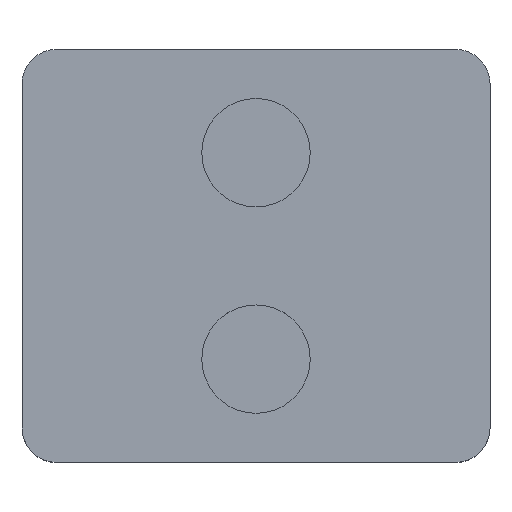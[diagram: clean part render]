
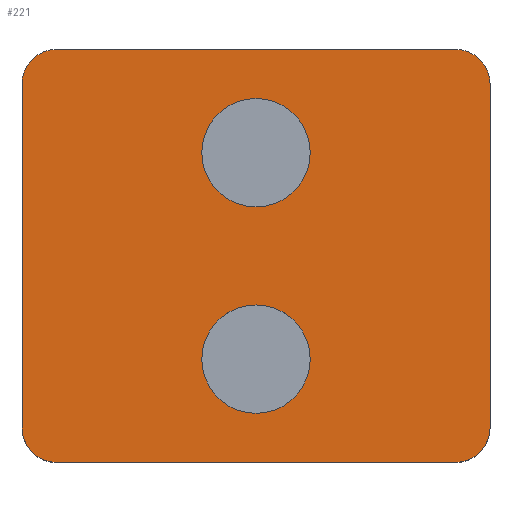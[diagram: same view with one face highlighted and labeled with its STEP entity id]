
A CAD part, top view. The second image highlights one B-rep face of the part: STEP entity #221.
In plain terms, the highlighted planar face has unit normal (0, 0, 1).
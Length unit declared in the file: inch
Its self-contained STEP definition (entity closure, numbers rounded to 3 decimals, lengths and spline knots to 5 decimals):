
#15=FACE_BOUND('',#42,.T.);
#16=FACE_BOUND('',#43,.T.);
#18=PLANE('',#251);
#27=FACE_OUTER_BOUND('',#41,.T.);
#41=EDGE_LOOP('',(#161,#162,#163,#164,#165,#166,#167,#168));
#42=EDGE_LOOP('',(#169));
#43=EDGE_LOOP('',(#170));
#57=LINE('',#357,#75);
#60=LINE('',#363,#78);
#61=LINE('',#367,#79);
#62=LINE('',#371,#80);
#75=VECTOR('',#285,0.3937);
#78=VECTOR('',#290,0.3937);
#79=VECTOR('',#293,0.3937);
#80=VECTOR('',#296,0.3937);
#92=CIRCLE('',#249,0.0625);
#93=CIRCLE('',#252,0.0625);
#94=CIRCLE('',#253,0.0625);
#95=CIRCLE('',#254,0.0625);
#96=CIRCLE('',#255,0.09843);
#97=CIRCLE('',#256,0.09843);
#105=VERTEX_POINT('',#350);
#106=VERTEX_POINT('',#352);
#107=VERTEX_POINT('',#356);
#109=VERTEX_POINT('',#362);
#110=VERTEX_POINT('',#364);
#111=VERTEX_POINT('',#366);
#112=VERTEX_POINT('',#368);
#113=VERTEX_POINT('',#370);
#114=VERTEX_POINT('',#373);
#115=VERTEX_POINT('',#375);
#125=EDGE_CURVE('',#105,#106,#92,.T.);
#127=EDGE_CURVE('',#107,#106,#57,.T.);
#130=EDGE_CURVE('',#105,#109,#60,.T.);
#131=EDGE_CURVE('',#110,#109,#93,.T.);
#132=EDGE_CURVE('',#110,#111,#61,.T.);
#133=EDGE_CURVE('',#112,#111,#94,.T.);
#134=EDGE_CURVE('',#112,#113,#62,.T.);
#135=EDGE_CURVE('',#107,#113,#95,.T.);
#136=EDGE_CURVE('',#114,#114,#96,.T.);
#137=EDGE_CURVE('',#115,#115,#97,.T.);
#161=ORIENTED_EDGE('',*,*,#125,.F.);
#162=ORIENTED_EDGE('',*,*,#130,.T.);
#163=ORIENTED_EDGE('',*,*,#131,.F.);
#164=ORIENTED_EDGE('',*,*,#132,.T.);
#165=ORIENTED_EDGE('',*,*,#133,.F.);
#166=ORIENTED_EDGE('',*,*,#134,.T.);
#167=ORIENTED_EDGE('',*,*,#135,.F.);
#168=ORIENTED_EDGE('',*,*,#127,.T.);
#169=ORIENTED_EDGE('',*,*,#136,.T.);
#170=ORIENTED_EDGE('',*,*,#137,.T.);
#221=ADVANCED_FACE('',(#27,#15,#16),#18,.T.);
#249=AXIS2_PLACEMENT_3D('',#353,#280,#281);
#251=AXIS2_PLACEMENT_3D('',#361,#288,#289);
#252=AXIS2_PLACEMENT_3D('',#365,#291,#292);
#253=AXIS2_PLACEMENT_3D('',#369,#294,#295);
#254=AXIS2_PLACEMENT_3D('',#372,#297,#298);
#255=AXIS2_PLACEMENT_3D('',#374,#299,#300);
#256=AXIS2_PLACEMENT_3D('',#376,#301,#302);
#280=DIRECTION('center_axis',(0.,0.,-1.));
#281=DIRECTION('ref_axis',(-0.707,0.707,0.));
#285=DIRECTION('',(-1.,0.,0.));
#288=DIRECTION('center_axis',(0.,0.,1.));
#289=DIRECTION('ref_axis',(1.,0.,0.));
#290=DIRECTION('',(0.,-1.,0.));
#291=DIRECTION('center_axis',(0.,0.,-1.));
#292=DIRECTION('ref_axis',(-0.707,-0.707,0.));
#293=DIRECTION('',(1.,0.,0.));
#294=DIRECTION('center_axis',(0.,0.,-1.));
#295=DIRECTION('ref_axis',(0.707,-0.707,0.));
#296=DIRECTION('',(0.,1.,0.));
#297=DIRECTION('center_axis',(0.,0.,-1.));
#298=DIRECTION('ref_axis',(0.707,0.707,0.));
#299=DIRECTION('center_axis',(0.,0.,-1.));
#300=DIRECTION('ref_axis',(1.,0.,0.));
#301=DIRECTION('center_axis',(0.,0.,-1.));
#302=DIRECTION('ref_axis',(1.,0.,0.));
#350=CARTESIAN_POINT('',(-9.83169,-1.33415,3.275));
#352=CARTESIAN_POINT('',(-9.76919,-1.27165,3.275));
#353=CARTESIAN_POINT('Origin',(-9.76919,-1.33415,3.275));
#356=CARTESIAN_POINT('',(-9.04419,-1.27165,3.275));
#357=CARTESIAN_POINT('',(-8.98169,-1.27165,3.275));
#361=CARTESIAN_POINT('Origin',(-9.40669,-1.64665,3.275));
#362=CARTESIAN_POINT('',(-9.83169,-1.95915,3.275));
#363=CARTESIAN_POINT('',(-9.83169,-1.27165,3.275));
#364=CARTESIAN_POINT('',(-9.76919,-2.02165,3.275));
#365=CARTESIAN_POINT('Origin',(-9.76919,-1.95915,3.275));
#366=CARTESIAN_POINT('',(-9.04419,-2.02165,3.275));
#367=CARTESIAN_POINT('',(-9.83169,-2.02165,3.275));
#368=CARTESIAN_POINT('',(-8.98169,-1.95915,3.275));
#369=CARTESIAN_POINT('Origin',(-9.04419,-1.95915,3.275));
#370=CARTESIAN_POINT('',(-8.98169,-1.33415,3.275));
#371=CARTESIAN_POINT('',(-8.98169,-2.02165,3.275));
#372=CARTESIAN_POINT('Origin',(-9.04419,-1.33415,3.275));
#373=CARTESIAN_POINT('',(-9.50512,-1.83415,3.275));
#374=CARTESIAN_POINT('Origin',(-9.40669,-1.83415,3.275));
#375=CARTESIAN_POINT('',(-9.50512,-1.45915,3.275));
#376=CARTESIAN_POINT('Origin',(-9.40669,-1.45915,3.275));
